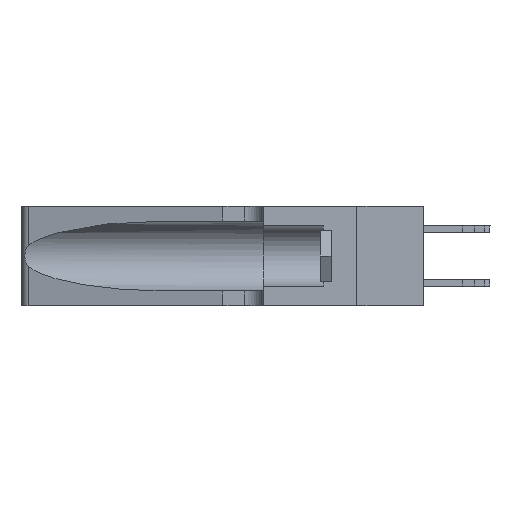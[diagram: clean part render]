
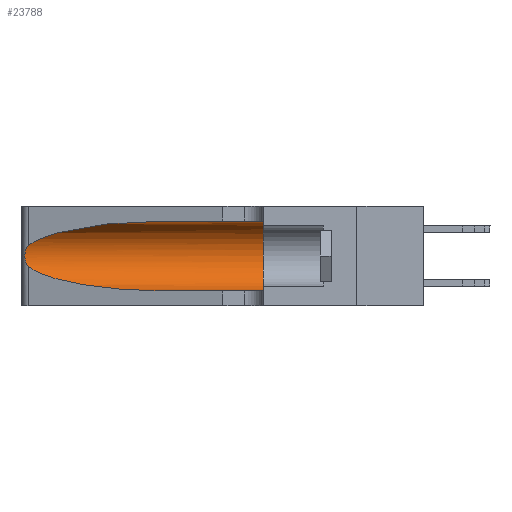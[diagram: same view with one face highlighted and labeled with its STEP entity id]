
A CAD part, left-side view. The second image highlights one B-rep face of the part: STEP entity #23788.
In plain terms, the highlighted cylindrical face has radius 3.308 mm (diameter 6.617 mm), a partial arc.
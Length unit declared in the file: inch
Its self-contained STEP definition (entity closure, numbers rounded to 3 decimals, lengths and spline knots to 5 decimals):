
#67 = VECTOR ( 'NONE', #8586, 39.37008 ) ;
#140 = CARTESIAN_POINT ( 'NONE',  ( 0.26018, 1.23835, 0.19895 ) ) ;
#1385 = CARTESIAN_POINT ( 'NONE',  ( 0.25487, 1.22718, 0.14631 ) ) ;
#1480 = CARTESIAN_POINT ( 'NONE',  ( 0.25487, 1.22718, 0.22369 ) ) ;
#2082 = VERTEX_POINT ( 'NONE', #19896 ) ;
#2292 = CARTESIAN_POINT ( 'NONE',  ( 0.1305, 0.72297, 0.31525 ) ) ;
#2393 = CARTESIAN_POINT ( 'NONE',  ( 0.18966, 0.96281, 0.31525 ) ) ;
#2729 = CARTESIAN_POINT ( 'NONE',  ( 0.25789, 1.23486, 0.15765 ) ) ;
#4975 = CARTESIAN_POINT ( 'NONE',  ( 0.1305, 0.35, 0.31525 ) ) ;
#5275 = VERTEX_POINT ( 'NONE', #1480 ) ;
#5572 = CYLINDRICAL_SURFACE ( 'NONE', #25166, 0.13025 ) ;
#6782 =( BOUNDED_CURVE ( )  B_SPLINE_CURVE ( 3, ( #2292, #2393, #12932, #28278 ),
 .UNSPECIFIED., .F., .T. ) 
 B_SPLINE_CURVE_WITH_KNOTS ( ( 4, 4 ),
 ( 1.5708, 2.84003 ),
 .UNSPECIFIED. ) 
 CURVE ( )  GEOMETRIC_REPRESENTATION_ITEM ( )  RATIONAL_B_SPLINE_CURVE ( ( 1., 0.87, 0.87, 1. ) ) 
 REPRESENTATION_ITEM ( '' )  );
#7629 = CARTESIAN_POINT ( 'NONE',  ( 0.25787, 1.23484, 0.2124 ) ) ;
#7728 = CARTESIAN_POINT ( 'NONE',  ( 0.25555, 1.22994, 0.2215 ) ) ;
#7871 = AXIS2_PLACEMENT_3D ( 'NONE', #15429, #10520, #23054 ) ;
#8586 = DIRECTION ( 'NONE',  ( 0., -1., 0. ) ) ;
#8753 = LINE ( 'NONE', #32143, #28019 ) ;
#9620 = ORIENTED_EDGE ( 'NONE', *, *, #17805, .T. ) ;
#10196 = CARTESIAN_POINT ( 'NONE',  ( 0.25639, 1.23184, 0.21858 ) ) ;
#10299 = CARTESIAN_POINT ( 'NONE',  ( 0.25555, 1.22993, 0.14849 ) ) ;
#10520 = DIRECTION ( 'NONE',  ( 0., 1., 0. ) ) ;
#10595 = CARTESIAN_POINT ( 'NONE',  ( 0.25854, 1.2359, 0.20912 ) ) ;
#10876 = VERTEX_POINT ( 'NONE', #4975 ) ;
#12922 = EDGE_CURVE ( 'NONE', #18959, #25802, #21703, .T. ) ;
#12932 = CARTESIAN_POINT ( 'NONE',  ( 0.2373, 1.15595, 0.28018 ) ) ;
#13027 = CIRCLE ( 'NONE', #7871, 0.13025 ) ;
#13156 = CARTESIAN_POINT ( 'NONE',  ( 0.26075, 1.23896, 0.19203 ) ) ;
#13585 = CARTESIAN_POINT ( 'NONE',  ( 0.25487, 1.22718, 0.14631 ) ) ;
#13741 = ORIENTED_EDGE ( 'NONE', *, *, #21116, .T. ) ;
#14762 = CARTESIAN_POINT ( 'NONE',  ( 0.26017, 1.23833, 0.17102 ) ) ;
#15429 = CARTESIAN_POINT ( 'NONE',  ( 0.1305, 0.35, 0.185 ) ) ;
#15555 = FACE_OUTER_BOUND ( 'NONE', #19474, .T. ) ;
#16456 = CARTESIAN_POINT ( 'NONE',  ( 0.1305, 0.72297, 0.05475 ) ) ;
#16922 = CARTESIAN_POINT ( 'NONE',  ( 0.25487, 1.22718, 0.14631 ) ) ;
#17000 = CARTESIAN_POINT ( 'NONE',  ( 0.1305, 0.35, 0.05475 ) ) ;
#17286 = EDGE_CURVE ( 'NONE', #10876, #20357, #13027, .T. ) ;
#17734 = ORIENTED_EDGE ( 'NONE', *, *, #29131, .T. ) ;
#17805 = EDGE_CURVE ( 'NONE', #5275, #18959, #27261, .T. ) ;
#17900 = ORIENTED_EDGE ( 'NONE', *, *, #17286, .F. ) ;
#18413 = DIRECTION ( 'NONE',  ( 0., 0., -1. ) ) ;
#18959 = VERTEX_POINT ( 'NONE', #16922 ) ;
#19474 = EDGE_LOOP ( 'NONE', ( #17734, #9620, #26551, #13741, #17900, #19617 ) ) ;
#19617 = ORIENTED_EDGE ( 'NONE', *, *, #20234, .F. ) ;
#19623 = LINE ( 'NONE', #29186, #67 ) ;
#19896 = CARTESIAN_POINT ( 'NONE',  ( 0.1305, 0.72297, 0.31525 ) ) ;
#19902 = CARTESIAN_POINT ( 'NONE',  ( 0.25639, 1.23186, 0.15144 ) ) ;
#20234 = EDGE_CURVE ( 'NONE', #2082, #10876, #19623, .T. ) ;
#20357 = VERTEX_POINT ( 'NONE', #17000 ) ;
#20655 = CARTESIAN_POINT ( 'NONE',  ( 0.25487, 1.22718, 0.22369 ) ) ;
#20778 = DIRECTION ( 'NONE',  ( 0., -1., 0. ) ) ;
#21116 = EDGE_CURVE ( 'NONE', #25802, #20357, #8753, .T. ) ;
#21472 = CARTESIAN_POINT ( 'NONE',  ( 0.2373, 1.15595, 0.08982 ) ) ;
#21703 =( BOUNDED_CURVE ( )  B_SPLINE_CURVE ( 3, ( #1385, #21472, #21930, #24372 ),
 .UNSPECIFIED., .F., .F. ) 
 B_SPLINE_CURVE_WITH_KNOTS ( ( 4, 4 ),
 ( 3.44316, 4.71239 ),
 .UNSPECIFIED. ) 
 CURVE ( )  GEOMETRIC_REPRESENTATION_ITEM ( )  RATIONAL_B_SPLINE_CURVE ( ( 1., 0.87, 0.87, 1. ) ) 
 REPRESENTATION_ITEM ( '' )  );
#21930 = CARTESIAN_POINT ( 'NONE',  ( 0.18966, 0.96281, 0.05475 ) ) ;
#23054 = DIRECTION ( 'NONE',  ( 0., 0., 1. ) ) ;
#23788 = ADVANCED_FACE ( 'NONE', ( #15555 ), #5572, .F. ) ;
#24372 = CARTESIAN_POINT ( 'NONE',  ( 0.1305, 0.72297, 0.05475 ) ) ;
#25166 = AXIS2_PLACEMENT_3D ( 'NONE', #31219, #20778, #18413 ) ;
#25260 = DIRECTION ( 'NONE',  ( 0., -1., 0. ) ) ;
#25599 = CARTESIAN_POINT ( 'NONE',  ( 0.26075, 1.23896, 0.178 ) ) ;
#25802 = VERTEX_POINT ( 'NONE', #16456 ) ;
#26551 = ORIENTED_EDGE ( 'NONE', *, *, #12922, .T. ) ;
#27261 = B_SPLINE_CURVE_WITH_KNOTS ( 'NONE', 3,
 ( #20655, #7728, #10196, #7629, #10595, #140, #13156, #25599, #14762, #32711, #2729, #19902, #10299, #13585 ),
 .UNSPECIFIED., .F., .F.,
 ( 4, 2, 2, 2, 2, 2, 4 ),
 ( 0., 0.00027, 0.00053, 0.00107, 0.0016, 0.00187, 0.00214 ),
 .UNSPECIFIED. ) ;
#28019 = VECTOR ( 'NONE', #25260, 39.37008 ) ;
#28278 = CARTESIAN_POINT ( 'NONE',  ( 0.25487, 1.22718, 0.22369 ) ) ;
#29131 = EDGE_CURVE ( 'NONE', #2082, #5275, #6782, .T. ) ;
#29186 = CARTESIAN_POINT ( 'NONE',  ( 0.1305, 1.61858, 0.31525 ) ) ;
#31219 = CARTESIAN_POINT ( 'NONE',  ( 0.1305, 1.61858, 0.185 ) ) ;
#32143 = CARTESIAN_POINT ( 'NONE',  ( 0.1305, 1.61858, 0.05475 ) ) ;
#32711 = CARTESIAN_POINT ( 'NONE',  ( 0.25856, 1.23593, 0.16098 ) ) ;
